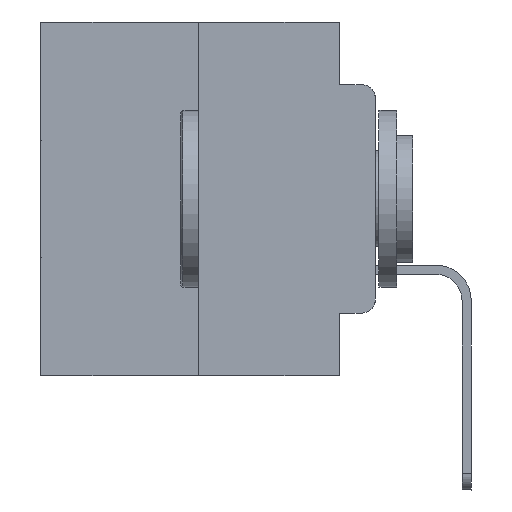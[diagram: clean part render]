
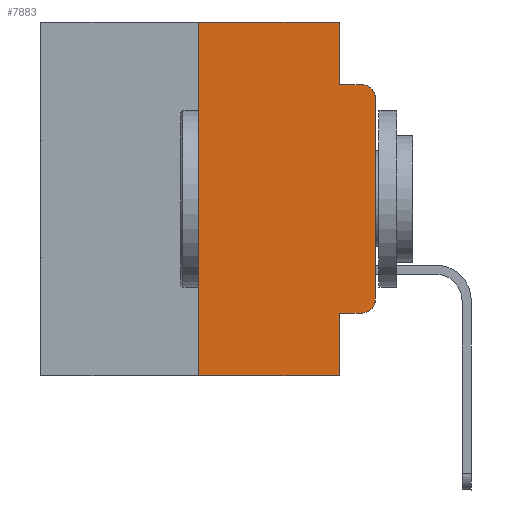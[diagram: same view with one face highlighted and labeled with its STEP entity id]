
A CAD part, left-side view. The second image highlights one B-rep face of the part: STEP entity #7883.
In plain terms, the highlighted planar face has unit normal (-1, 0, 0).
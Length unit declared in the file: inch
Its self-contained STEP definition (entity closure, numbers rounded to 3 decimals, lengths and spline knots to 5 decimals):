
#4 = VECTOR ( 'NONE', #5302, 39.37008 ) ;
#396 = LINE ( 'NONE', #20834, #16789 ) ;
#407 = CARTESIAN_POINT ( 'NONE',  ( 0., 0.473, 0. ) ) ;
#436 = ORIENTED_EDGE ( 'NONE', *, *, #21172, .F. ) ;
#470 = EDGE_CURVE ( 'NONE', #22380, #13374, #8714, .T. ) ;
#519 = AXIS2_PLACEMENT_3D ( 'NONE', #15539, #6987, #15359 ) ;
#582 = ORIENTED_EDGE ( 'NONE', *, *, #14670, .T. ) ;
#613 = DIRECTION ( 'NONE',  ( 0., -1., 0. ) ) ;
#788 = ORIENTED_EDGE ( 'NONE', *, *, #1077, .T. ) ;
#874 = VECTOR ( 'NONE', #4898, 39.37008 ) ;
#1077 = EDGE_CURVE ( 'NONE', #19944, #25156, #24649, .T. ) ;
#1164 = VERTEX_POINT ( 'NONE', #10483 ) ;
#1280 = DIRECTION ( 'NONE',  ( 0., 0., 1. ) ) ;
#1296 = CARTESIAN_POINT ( 'NONE',  ( 0., 0.051, -0.0885 ) ) ;
#1447 = DIRECTION ( 'NONE',  ( 0., 0., -1. ) ) ;
#2777 = AXIS2_PLACEMENT_3D ( 'NONE', #9352, #17943, #13633 ) ;
#3250 = LINE ( 'NONE', #407, #7292 ) ;
#3333 = DIRECTION ( 'NONE',  ( 0., 0., -1. ) ) ;
#4780 = VERTEX_POINT ( 'NONE', #17571 ) ;
#4898 = DIRECTION ( 'NONE',  ( 0., 0., -1. ) ) ;
#5302 = DIRECTION ( 'NONE',  ( 0., -1., 0. ) ) ;
#6362 = AXIS2_PLACEMENT_3D ( 'NONE', #12102, #27000, #1447 ) ;
#6474 = CARTESIAN_POINT ( 'NONE',  ( 0., 0., -0.3915 ) ) ;
#6856 = CARTESIAN_POINT ( 'NONE',  ( 0., 0.02, -0.4115 ) ) ;
#6980 = LINE ( 'NONE', #11249, #20322 ) ;
#6987 = DIRECTION ( 'NONE',  ( 1., 0., 0. ) ) ;
#7292 = VECTOR ( 'NONE', #19620, 39.37008 ) ;
#7525 = EDGE_CURVE ( 'NONE', #14551, #19944, #7790, .T. ) ;
#7790 = LINE ( 'NONE', #22155, #14757 ) ;
#7883 = ADVANCED_FACE ( 'NONE', ( #21084 ), #13315, .F. ) ;
#7989 = DIRECTION ( 'NONE',  ( 0., 0., 1. ) ) ;
#8273 = EDGE_LOOP ( 'NONE', ( #11974, #12964, #20605, #20494, #23806, #21293, #582, #436, #18941, #788 ) ) ;
#8714 = LINE ( 'NONE', #1296, #4 ) ;
#9352 = CARTESIAN_POINT ( 'NONE',  ( 0., 0.02, -0.1085 ) ) ;
#10483 = CARTESIAN_POINT ( 'NONE',  ( 0., 0.051, -0.5 ) ) ;
#11249 = CARTESIAN_POINT ( 'NONE',  ( 0., 0.473, -0.5 ) ) ;
#11974 = ORIENTED_EDGE ( 'NONE', *, *, #17080, .T. ) ;
#12001 = EDGE_CURVE ( 'NONE', #18707, #4780, #396, .T. ) ;
#12102 = CARTESIAN_POINT ( 'NONE',  ( 0., 0.02, -0.3915 ) ) ;
#12246 = LINE ( 'NONE', #13397, #874 ) ;
#12482 = VERTEX_POINT ( 'NONE', #19960 ) ;
#12964 = ORIENTED_EDGE ( 'NONE', *, *, #23459, .T. ) ;
#13315 = PLANE ( 'NONE',  #519 ) ;
#13374 = VERTEX_POINT ( 'NONE', #21652 ) ;
#13397 = CARTESIAN_POINT ( 'NONE',  ( 0., 0.051, 0. ) ) ;
#13425 = CARTESIAN_POINT ( 'NONE',  ( 0., 0.25, -0.5 ) ) ;
#13633 = DIRECTION ( 'NONE',  ( 0., 0., -1. ) ) ;
#14137 = CARTESIAN_POINT ( 'NONE',  ( 0., 0.051, 0. ) ) ;
#14151 = VECTOR ( 'NONE', #1280, 39.37008 ) ;
#14473 = LINE ( 'NONE', #20408, #14151 ) ;
#14551 = VERTEX_POINT ( 'NONE', #21230 ) ;
#14670 = EDGE_CURVE ( 'NONE', #18707, #1164, #6980, .T. ) ;
#14757 = VECTOR ( 'NONE', #26380, 39.37008 ) ;
#14763 = EDGE_CURVE ( 'NONE', #20417, #22380, #16301, .T. ) ;
#15169 = EDGE_CURVE ( 'NONE', #4780, #20417, #3250, .T. ) ;
#15359 = DIRECTION ( 'NONE',  ( 0., 0., -1. ) ) ;
#15539 = CARTESIAN_POINT ( 'NONE',  ( 0., 0.473, 0. ) ) ;
#16301 = LINE ( 'NONE', #14137, #21617 ) ;
#16789 = VECTOR ( 'NONE', #7989, 39.37008 ) ;
#16817 = CIRCLE ( 'NONE', #2777, 0.02 ) ;
#17080 = EDGE_CURVE ( 'NONE', #25156, #12482, #14473, .T. ) ;
#17571 = CARTESIAN_POINT ( 'NONE',  ( 0., 0.25, 0. ) ) ;
#17943 = DIRECTION ( 'NONE',  ( -1., 0., 0. ) ) ;
#18707 = VERTEX_POINT ( 'NONE', #13425 ) ;
#18941 = ORIENTED_EDGE ( 'NONE', *, *, #7525, .T. ) ;
#19620 = DIRECTION ( 'NONE',  ( 0., -1., 0. ) ) ;
#19944 = VERTEX_POINT ( 'NONE', #6856 ) ;
#19960 = CARTESIAN_POINT ( 'NONE',  ( 0., 0., -0.1085 ) ) ;
#20322 = VECTOR ( 'NONE', #613, 39.37008 ) ;
#20408 = CARTESIAN_POINT ( 'NONE',  ( 0., 0., 0. ) ) ;
#20417 = VERTEX_POINT ( 'NONE', #21714 ) ;
#20494 = ORIENTED_EDGE ( 'NONE', *, *, #14763, .F. ) ;
#20605 = ORIENTED_EDGE ( 'NONE', *, *, #470, .F. ) ;
#20834 = CARTESIAN_POINT ( 'NONE',  ( 0., 0.25, 0. ) ) ;
#21084 = FACE_OUTER_BOUND ( 'NONE', #8273, .T. ) ;
#21172 = EDGE_CURVE ( 'NONE', #14551, #1164, #12246, .T. ) ;
#21230 = CARTESIAN_POINT ( 'NONE',  ( 0., 0.051, -0.4115 ) ) ;
#21293 = ORIENTED_EDGE ( 'NONE', *, *, #12001, .F. ) ;
#21617 = VECTOR ( 'NONE', #3333, 39.37008 ) ;
#21652 = CARTESIAN_POINT ( 'NONE',  ( 0., 0.02, -0.0885 ) ) ;
#21714 = CARTESIAN_POINT ( 'NONE',  ( 0., 0.051, 0. ) ) ;
#22155 = CARTESIAN_POINT ( 'NONE',  ( 0., 0.051, -0.4115 ) ) ;
#22380 = VERTEX_POINT ( 'NONE', #24588 ) ;
#23459 = EDGE_CURVE ( 'NONE', #12482, #13374, #16817, .T. ) ;
#23806 = ORIENTED_EDGE ( 'NONE', *, *, #15169, .F. ) ;
#24588 = CARTESIAN_POINT ( 'NONE',  ( 0., 0.051, -0.0885 ) ) ;
#24649 = CIRCLE ( 'NONE', #6362, 0.02 ) ;
#25156 = VERTEX_POINT ( 'NONE', #6474 ) ;
#26380 = DIRECTION ( 'NONE',  ( 0., -1., 0. ) ) ;
#27000 = DIRECTION ( 'NONE',  ( -1., 0., 0. ) ) ;
